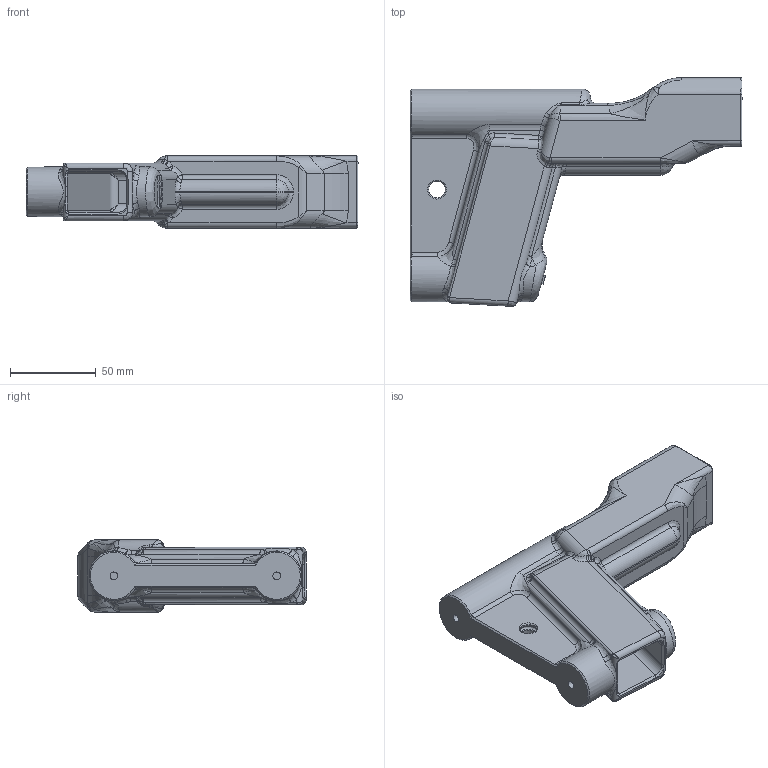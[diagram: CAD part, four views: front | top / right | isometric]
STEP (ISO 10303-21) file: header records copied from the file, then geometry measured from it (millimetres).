
FILE_DESCRIPTION (( 'STEP AP203' ), '1' );
FILE_NAME ('WTF-9_stock.STEP', '2020-05-09T10:05:50', ( '' ), ( '' ), 'SwSTEP 2.0', 'SolidWorks 2016', '' );
FILE_SCHEMA (( 'CONFIG_CONTROL_DESIGN' ));
Length unit declared in the file: millimetre
Products named in the file (2): WTF-9_stock; WTF9 V1 FINAL_21
Assembly tree (1 placements, depth 2):
  WTF-9_stock
    WTF9 V1 FINAL_21
Bounding box: 193.67 x 133.37 x 42 mm (x, y, z)
Surface area: 62685.2 mm2 (no closed solid volume)
Topology: 0 solids, 1 shells, 367 faces, 900 edges, 523 vertices
Faces by surface type: bspline 158, plane 109, cylinder 92, cone 8
Full cylindrical faces by diameter (mm): 4.5 x2, 9.6 x2
Entity records: 18248 total; most frequent: CARTESIAN_POINT 11066, ORIENTED_EDGE 1713, DIRECTION 941, EDGE_CURVE 861, VERTEX_POINT 511, B_SPLINE_CURVE_WITH_KNOTS 401, EDGE_LOOP 385, FACE_OUTER_BOUND 378
